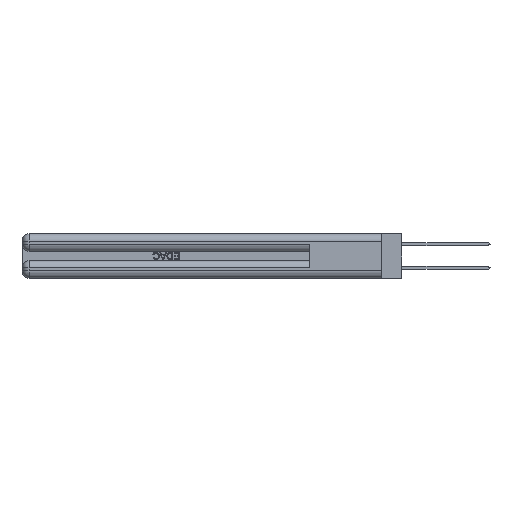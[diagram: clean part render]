
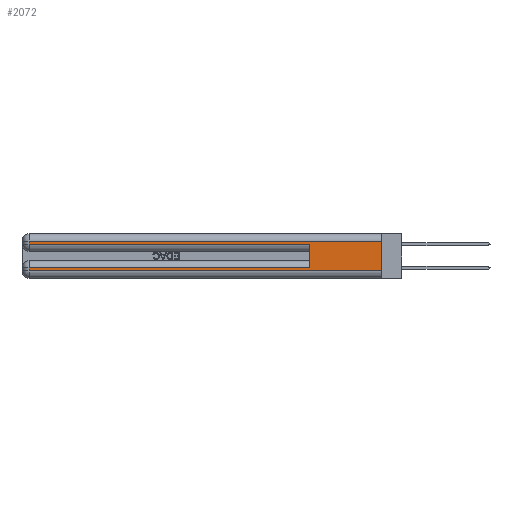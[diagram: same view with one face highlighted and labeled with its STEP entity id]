
A CAD part, left-side view. The second image highlights one B-rep face of the part: STEP entity #2072.
In plain terms, the highlighted planar face has unit normal (-1, 0, 0).
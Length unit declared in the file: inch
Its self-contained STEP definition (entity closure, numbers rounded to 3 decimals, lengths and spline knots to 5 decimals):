
#113 = CARTESIAN_POINT ( 'NONE',  ( 0., 0., 0.37 ) ) ;
#994 = CARTESIAN_POINT ( 'NONE',  ( 0., 0., 0.31 ) ) ;
#1437 = CARTESIAN_POINT ( 'NONE',  ( 0., 0., 0.31 ) ) ;
#2072 = ADVANCED_FACE ( 'NONE', ( #27300 ), #12452, .F. ) ;
#2672 = VECTOR ( 'NONE', #10511, 39.37008 ) ;
#3570 = ORIENTED_EDGE ( 'NONE', *, *, #37334, .F. ) ;
#4064 = EDGE_CURVE ( 'NONE', #22282, #27204, #16840, .T. ) ;
#5557 = ORIENTED_EDGE ( 'NONE', *, *, #16353, .T. ) ;
#5787 = VECTOR ( 'NONE', #6028, 39.37008 ) ;
#6028 = DIRECTION ( 'NONE',  ( 0., -1., 0. ) ) ;
#6637 = DIRECTION ( 'NONE',  ( 0., 0., -1. ) ) ;
#8783 = VERTEX_POINT ( 'NONE', #40161 ) ;
#9048 = CARTESIAN_POINT ( 'NONE',  ( 0., 0., 0.37 ) ) ;
#10101 = EDGE_CURVE ( 'NONE', #14509, #33027, #18564, .T. ) ;
#10438 = CARTESIAN_POINT ( 'NONE',  ( 0., 0., 0.06 ) ) ;
#10511 = DIRECTION ( 'NONE',  ( 0., 0., 1. ) ) ;
#10956 = VECTOR ( 'NONE', #23803, 39.37008 ) ;
#11469 = CARTESIAN_POINT ( 'NONE',  ( 0., 2.94, 0.085 ) ) ;
#12050 = ORIENTED_EDGE ( 'NONE', *, *, #27176, .T. ) ;
#12452 = PLANE ( 'NONE',  #33715 ) ;
#12779 = LINE ( 'NONE', #33615, #29696 ) ;
#12951 = ORIENTED_EDGE ( 'NONE', *, *, #4064, .T. ) ;
#13852 = DIRECTION ( 'NONE',  ( 0., -1., 0. ) ) ;
#14508 = LINE ( 'NONE', #34205, #30352 ) ;
#14509 = VERTEX_POINT ( 'NONE', #17847 ) ;
#15875 = DIRECTION ( 'NONE',  ( 0., 0., -1. ) ) ;
#16144 = EDGE_CURVE ( 'NONE', #8783, #34913, #12779, .T. ) ;
#16353 = EDGE_CURVE ( 'NONE', #14509, #31447, #42751, .T. ) ;
#16686 = ORIENTED_EDGE ( 'NONE', *, *, #27059, .T. ) ;
#16840 = LINE ( 'NONE', #10438, #33658 ) ;
#17167 = VECTOR ( 'NONE', #38120, 39.37008 ) ;
#17847 = CARTESIAN_POINT ( 'NONE',  ( 0., 0.6, 0.085 ) ) ;
#18499 = ORIENTED_EDGE ( 'NONE', *, *, #23451, .T. ) ;
#18564 = LINE ( 'NONE', #30746, #2672 ) ;
#21559 = CARTESIAN_POINT ( 'NONE',  ( 0., 0., 0.06 ) ) ;
#22282 = VERTEX_POINT ( 'NONE', #43061 ) ;
#22893 = CARTESIAN_POINT ( 'NONE',  ( 0., 0., 0.285 ) ) ;
#23205 = VERTEX_POINT ( 'NONE', #1437 ) ;
#23451 = EDGE_CURVE ( 'NONE', #34913, #33027, #23796, .T. ) ;
#23796 = LINE ( 'NONE', #22893, #5787 ) ;
#23803 = DIRECTION ( 'NONE',  ( 0., 0., -1. ) ) ;
#27059 = EDGE_CURVE ( 'NONE', #31447, #22282, #14508, .T. ) ;
#27176 = EDGE_CURVE ( 'NONE', #23205, #8783, #36096, .T. ) ;
#27204 = VERTEX_POINT ( 'NONE', #21559 ) ;
#27300 = FACE_OUTER_BOUND ( 'NONE', #29386, .T. ) ;
#27902 = LINE ( 'NONE', #113, #10956 ) ;
#29386 = EDGE_LOOP ( 'NONE', ( #3570, #12050, #34698, #18499, #39468, #5557, #16686, #12951 ) ) ;
#29696 = VECTOR ( 'NONE', #6637, 39.37008 ) ;
#30352 = VECTOR ( 'NONE', #40867, 39.37008 ) ;
#30746 = CARTESIAN_POINT ( 'NONE',  ( 0., 0.6, 0.145 ) ) ;
#31249 = DIRECTION ( 'NONE',  ( 0., 1., 0. ) ) ;
#31447 = VERTEX_POINT ( 'NONE', #11469 ) ;
#33027 = VERTEX_POINT ( 'NONE', #37318 ) ;
#33615 = CARTESIAN_POINT ( 'NONE',  ( 0., 2.94, 0.37 ) ) ;
#33658 = VECTOR ( 'NONE', #13852, 39.37008 ) ;
#33715 = AXIS2_PLACEMENT_3D ( 'NONE', #9048, #36026, #15875 ) ;
#33953 = VECTOR ( 'NONE', #31249, 39.37008 ) ;
#34205 = CARTESIAN_POINT ( 'NONE',  ( 0., 2.94, 0.37 ) ) ;
#34698 = ORIENTED_EDGE ( 'NONE', *, *, #16144, .T. ) ;
#34913 = VERTEX_POINT ( 'NONE', #40610 ) ;
#36026 = DIRECTION ( 'NONE',  ( 1., 0., 0. ) ) ;
#36096 = LINE ( 'NONE', #994, #17167 ) ;
#37318 = CARTESIAN_POINT ( 'NONE',  ( 0., 0.6, 0.285 ) ) ;
#37334 = EDGE_CURVE ( 'NONE', #23205, #27204, #27902, .T. ) ;
#37958 = CARTESIAN_POINT ( 'NONE',  ( 0., 0., 0.085 ) ) ;
#38120 = DIRECTION ( 'NONE',  ( 0., 1., 0. ) ) ;
#39468 = ORIENTED_EDGE ( 'NONE', *, *, #10101, .F. ) ;
#40161 = CARTESIAN_POINT ( 'NONE',  ( 0., 2.94, 0.31 ) ) ;
#40610 = CARTESIAN_POINT ( 'NONE',  ( 0., 2.94, 0.285 ) ) ;
#40867 = DIRECTION ( 'NONE',  ( 0., 0., -1. ) ) ;
#42751 = LINE ( 'NONE', #37958, #33953 ) ;
#43061 = CARTESIAN_POINT ( 'NONE',  ( 0., 2.94, 0.06 ) ) ;
